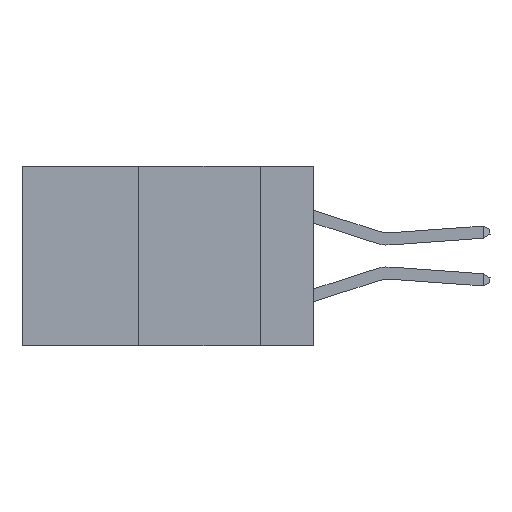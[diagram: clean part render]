
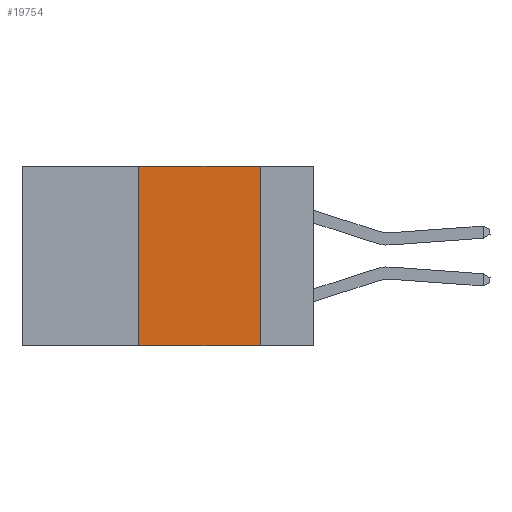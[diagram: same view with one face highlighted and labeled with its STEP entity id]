
A CAD part, left-side view. The second image highlights one B-rep face of the part: STEP entity #19754.
In plain terms, the highlighted planar face has unit normal (-1, 0, 0).
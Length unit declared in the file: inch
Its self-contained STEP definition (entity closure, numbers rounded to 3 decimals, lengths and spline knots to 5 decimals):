
#1261 = EDGE_CURVE ( 'NONE', #6363, #3681, #15131, .T. ) ;
#1539 = CARTESIAN_POINT ( 'NONE',  ( 0., 0.36, 0. ) ) ;
#3681 = VERTEX_POINT ( 'NONE', #20487 ) ;
#5906 = CARTESIAN_POINT ( 'NONE',  ( 0., 0.6, 0. ) ) ;
#6363 = VERTEX_POINT ( 'NONE', #19576 ) ;
#7136 = VECTOR ( 'NONE', #17649, 39.37008 ) ;
#9142 = DIRECTION ( 'NONE',  ( 1., 0., 0. ) ) ;
#9308 = VERTEX_POINT ( 'NONE', #10750 ) ;
#9776 = ORIENTED_EDGE ( 'NONE', *, *, #19679, .T. ) ;
#9869 = LINE ( 'NONE', #23833, #36708 ) ;
#10008 = EDGE_LOOP ( 'NONE', ( #22674, #25563, #34058, #9776 ) ) ;
#10750 = CARTESIAN_POINT ( 'NONE',  ( 0., 0.36, -0.37 ) ) ;
#14876 = AXIS2_PLACEMENT_3D ( 'NONE', #33492, #9142, #15301 ) ;
#15041 = PLANE ( 'NONE',  #14876 ) ;
#15131 = LINE ( 'NONE', #5906, #7136 ) ;
#15301 = DIRECTION ( 'NONE',  ( 0., 0., -1. ) ) ;
#16391 = LINE ( 'NONE', #22683, #34336 ) ;
#17562 = DIRECTION ( 'NONE',  ( 0., -1., 0. ) ) ;
#17649 = DIRECTION ( 'NONE',  ( 0., -1., 0. ) ) ;
#19576 = CARTESIAN_POINT ( 'NONE',  ( 0., 0.36, 0. ) ) ;
#19634 = VECTOR ( 'NONE', #25620, 39.37008 ) ;
#19679 = EDGE_CURVE ( 'NONE', #9308, #32975, #9869, .T. ) ;
#19754 = ADVANCED_FACE ( 'NONE', ( #26326 ), #15041, .F. ) ;
#20487 = CARTESIAN_POINT ( 'NONE',  ( 0., 0.11, 0. ) ) ;
#21509 = LINE ( 'NONE', #1539, #19634 ) ;
#22674 = ORIENTED_EDGE ( 'NONE', *, *, #34416, .F. ) ;
#22683 = CARTESIAN_POINT ( 'NONE',  ( 0., 0.11, 0. ) ) ;
#23833 = CARTESIAN_POINT ( 'NONE',  ( 0., 0.6, -0.37 ) ) ;
#24781 = EDGE_CURVE ( 'NONE', #9308, #6363, #21509, .T. ) ;
#25563 = ORIENTED_EDGE ( 'NONE', *, *, #1261, .F. ) ;
#25620 = DIRECTION ( 'NONE',  ( 0., 0., 1. ) ) ;
#26326 = FACE_OUTER_BOUND ( 'NONE', #10008, .T. ) ;
#31427 = DIRECTION ( 'NONE',  ( 0., 0., -1. ) ) ;
#31794 = CARTESIAN_POINT ( 'NONE',  ( 0., 0.11, -0.37 ) ) ;
#32975 = VERTEX_POINT ( 'NONE', #31794 ) ;
#33492 = CARTESIAN_POINT ( 'NONE',  ( 0., 0.6, 0. ) ) ;
#34058 = ORIENTED_EDGE ( 'NONE', *, *, #24781, .F. ) ;
#34336 = VECTOR ( 'NONE', #31427, 39.37008 ) ;
#34416 = EDGE_CURVE ( 'NONE', #3681, #32975, #16391, .T. ) ;
#36708 = VECTOR ( 'NONE', #17562, 39.37008 ) ;
